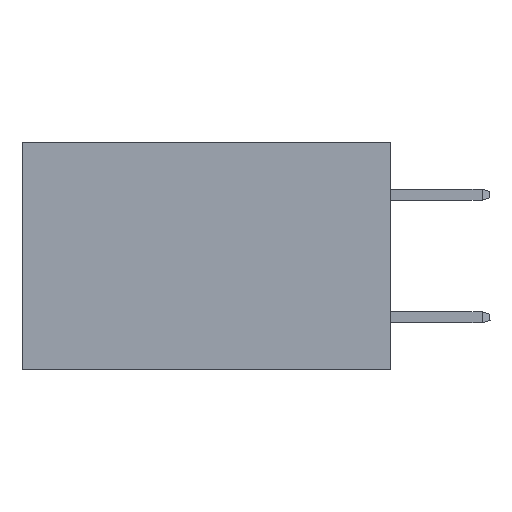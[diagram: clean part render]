
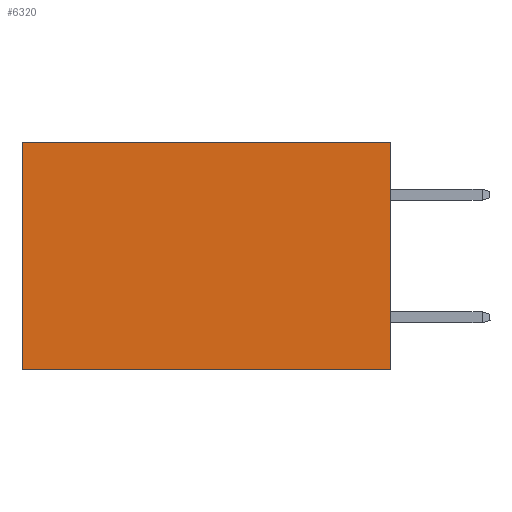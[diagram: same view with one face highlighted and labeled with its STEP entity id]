
A CAD part, left-side view. The second image highlights one B-rep face of the part: STEP entity #6320.
In plain terms, the highlighted planar face has unit normal (-1, 0, 0).
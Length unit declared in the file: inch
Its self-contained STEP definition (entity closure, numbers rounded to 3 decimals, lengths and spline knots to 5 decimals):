
#757 = LINE ( 'NONE', #3205, #5385 ) ;
#922 = DIRECTION ( 'NONE',  ( 0., 1., 0. ) ) ;
#1333 = CARTESIAN_POINT ( 'NONE',  ( 0.2875, 0., 0. ) ) ;
#1547 = VECTOR ( 'NONE', #8652, 39.37008 ) ;
#2143 = CARTESIAN_POINT ( 'NONE',  ( 0.2875, 0., -0.37 ) ) ;
#2476 = ORIENTED_EDGE ( 'NONE', *, *, #2805, .T. ) ;
#2490 = VERTEX_POINT ( 'NONE', #1333 ) ;
#2666 = AXIS2_PLACEMENT_3D ( 'NONE', #8577, #9079, #9566 ) ;
#2805 = EDGE_CURVE ( 'NONE', #2490, #10509, #757, .T. ) ;
#3129 = VECTOR ( 'NONE', #10088, 39.37008 ) ;
#3205 = CARTESIAN_POINT ( 'NONE',  ( 0.2875, 0., 0. ) ) ;
#3233 = VERTEX_POINT ( 'NONE', #10069 ) ;
#3678 = EDGE_CURVE ( 'NONE', #10509, #3233, #4473, .T. ) ;
#3889 = CARTESIAN_POINT ( 'NONE',  ( 0.2875, 0.6, 0. ) ) ;
#3912 = LINE ( 'NONE', #6019, #1547 ) ;
#3935 = DIRECTION ( 'NONE',  ( 0., 0., -1. ) ) ;
#4037 = CARTESIAN_POINT ( 'NONE',  ( 0.2875, 0.6, 0. ) ) ;
#4473 = LINE ( 'NONE', #4037, #7732 ) ;
#4578 = EDGE_LOOP ( 'NONE', ( #7992, #6117, #8718, #2476 ) ) ;
#4630 = EDGE_CURVE ( 'NONE', #2490, #9301, #7220, .T. ) ;
#5385 = VECTOR ( 'NONE', #922, 39.37008 ) ;
#6019 = CARTESIAN_POINT ( 'NONE',  ( 0.2875, 0., -0.37 ) ) ;
#6117 = ORIENTED_EDGE ( 'NONE', *, *, #6473, .F. ) ;
#6320 = ADVANCED_FACE ( 'NONE', ( #9645 ), #8322, .F. ) ;
#6473 = EDGE_CURVE ( 'NONE', #9301, #3233, #3912, .T. ) ;
#7220 = LINE ( 'NONE', #10476, #3129 ) ;
#7732 = VECTOR ( 'NONE', #3935, 39.37008 ) ;
#7992 = ORIENTED_EDGE ( 'NONE', *, *, #3678, .T. ) ;
#8322 = PLANE ( 'NONE',  #2666 ) ;
#8577 = CARTESIAN_POINT ( 'NONE',  ( 0.2875, 0., 0. ) ) ;
#8652 = DIRECTION ( 'NONE',  ( 0., 1., 0. ) ) ;
#8718 = ORIENTED_EDGE ( 'NONE', *, *, #4630, .F. ) ;
#9079 = DIRECTION ( 'NONE',  ( 1., 0., 0. ) ) ;
#9301 = VERTEX_POINT ( 'NONE', #2143 ) ;
#9566 = DIRECTION ( 'NONE',  ( 0., 0., -1. ) ) ;
#9645 = FACE_OUTER_BOUND ( 'NONE', #4578, .T. ) ;
#10069 = CARTESIAN_POINT ( 'NONE',  ( 0.2875, 0.6, -0.37 ) ) ;
#10088 = DIRECTION ( 'NONE',  ( 0., 0., -1. ) ) ;
#10476 = CARTESIAN_POINT ( 'NONE',  ( 0.2875, 0., 0. ) ) ;
#10509 = VERTEX_POINT ( 'NONE', #3889 ) ;
